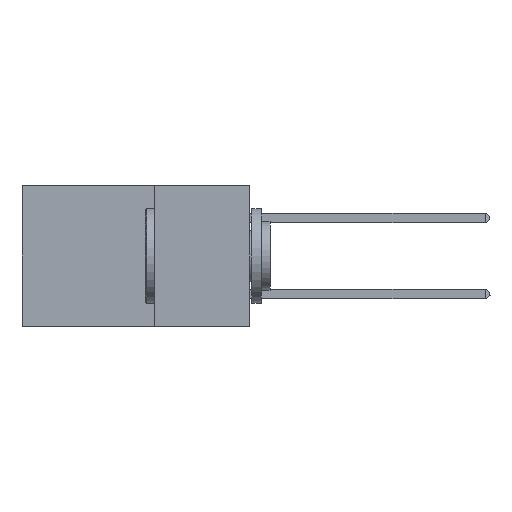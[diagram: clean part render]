
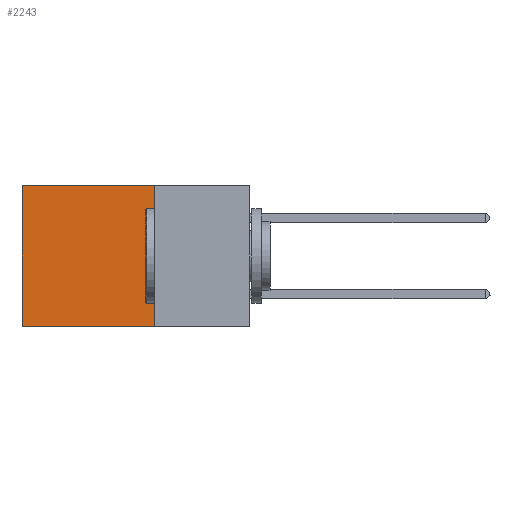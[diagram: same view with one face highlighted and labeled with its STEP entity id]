
A CAD part, left-side view. The second image highlights one B-rep face of the part: STEP entity #2243.
In plain terms, the highlighted planar face has unit normal (-1, 0, 0).
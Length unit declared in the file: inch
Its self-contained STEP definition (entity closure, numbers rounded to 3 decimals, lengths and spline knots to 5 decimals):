
#119 = CARTESIAN_POINT ( 'NONE',  ( 0.2875, 0.6, 0. ) ) ;
#1372 = EDGE_CURVE ( 'NONE', #11655, #10365, #17672, .T. ) ;
#1410 = ORIENTED_EDGE ( 'NONE', *, *, #1372, .F. ) ;
#1789 = DIRECTION ( 'NONE',  ( 0., 0., -1. ) ) ;
#2243 = ADVANCED_FACE ( 'NONE', ( #16358 ), #8964, .F. ) ;
#3331 = VECTOR ( 'NONE', #1789, 39.37008 ) ;
#3947 = VECTOR ( 'NONE', #15495, 39.37008 ) ;
#5885 = VERTEX_POINT ( 'NONE', #23383 ) ;
#6804 = DIRECTION ( 'NONE',  ( 1., 0., 0. ) ) ;
#6864 = CARTESIAN_POINT ( 'NONE',  ( 0.2875, 0.25, -0.37 ) ) ;
#7536 = LINE ( 'NONE', #20857, #8523 ) ;
#7841 = ORIENTED_EDGE ( 'NONE', *, *, #22710, .T. ) ;
#8337 = CARTESIAN_POINT ( 'NONE',  ( 0.2875, 0.6, 0. ) ) ;
#8523 = VECTOR ( 'NONE', #20599, 39.37008 ) ;
#8964 = PLANE ( 'NONE',  #21953 ) ;
#9047 = CARTESIAN_POINT ( 'NONE',  ( 0.2875, 0.25, -0.37 ) ) ;
#9629 = VERTEX_POINT ( 'NONE', #8337 ) ;
#10365 = VERTEX_POINT ( 'NONE', #14830 ) ;
#10488 = EDGE_LOOP ( 'NONE', ( #7841, #1410, #11095, #24982 ) ) ;
#11095 = ORIENTED_EDGE ( 'NONE', *, *, #15452, .F. ) ;
#11655 = VERTEX_POINT ( 'NONE', #9047 ) ;
#12269 = LINE ( 'NONE', #26315, #3331 ) ;
#13103 = CARTESIAN_POINT ( 'NONE',  ( 0.2875, 0.25, 0. ) ) ;
#14830 = CARTESIAN_POINT ( 'NONE',  ( 0.2875, 0.6, -0.37 ) ) ;
#15452 = EDGE_CURVE ( 'NONE', #5885, #11655, #12269, .T. ) ;
#15495 = DIRECTION ( 'NONE',  ( 0., 1., 0. ) ) ;
#16358 = FACE_OUTER_BOUND ( 'NONE', #10488, .T. ) ;
#17672 = LINE ( 'NONE', #6864, #3947 ) ;
#20599 = DIRECTION ( 'NONE',  ( 0., 1., 0. ) ) ;
#20857 = CARTESIAN_POINT ( 'NONE',  ( 0.2875, 0.25, 0. ) ) ;
#21953 = AXIS2_PLACEMENT_3D ( 'NONE', #13103, #6804, #23295 ) ;
#22033 = VECTOR ( 'NONE', #24523, 39.37008 ) ;
#22690 = LINE ( 'NONE', #119, #22033 ) ;
#22710 = EDGE_CURVE ( 'NONE', #9629, #10365, #22690, .T. ) ;
#23295 = DIRECTION ( 'NONE',  ( 0., 0., -1. ) ) ;
#23383 = CARTESIAN_POINT ( 'NONE',  ( 0.2875, 0.25, 0. ) ) ;
#24438 = EDGE_CURVE ( 'NONE', #5885, #9629, #7536, .T. ) ;
#24523 = DIRECTION ( 'NONE',  ( 0., 0., -1. ) ) ;
#24982 = ORIENTED_EDGE ( 'NONE', *, *, #24438, .T. ) ;
#26315 = CARTESIAN_POINT ( 'NONE',  ( 0.2875, 0.25, 0. ) ) ;
